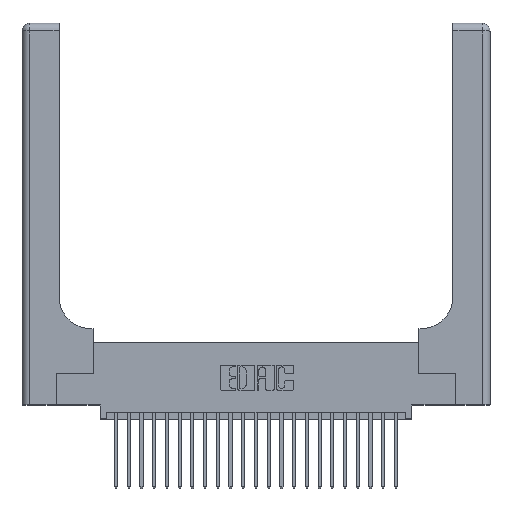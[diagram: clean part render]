
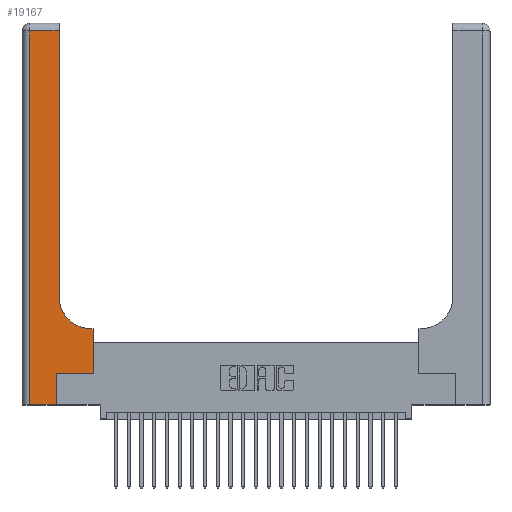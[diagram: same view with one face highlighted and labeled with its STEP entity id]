
A CAD part, top view. The second image highlights one B-rep face of the part: STEP entity #19167.
In plain terms, the highlighted planar face has unit normal (0, 0, 1).
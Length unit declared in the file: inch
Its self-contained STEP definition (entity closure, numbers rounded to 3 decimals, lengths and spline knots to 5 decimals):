
#268 = DIRECTION ( 'NONE',  ( -1., 0., 0. ) ) ;
#903 = VERTEX_POINT ( 'NONE', #4568 ) ;
#932 = ORIENTED_EDGE ( 'NONE', *, *, #19838, .T. ) ;
#1337 = CARTESIAN_POINT ( 'NONE',  ( 0.2915, 3., 0.37 ) ) ;
#1704 = EDGE_CURVE ( 'NONE', #14161, #14993, #12428, .T. ) ;
#1859 = VERTEX_POINT ( 'NONE', #20429 ) ;
#2014 = VECTOR ( 'NONE', #23446, 39.37008 ) ;
#2452 = VECTOR ( 'NONE', #6603, 39.37008 ) ;
#2461 = EDGE_CURVE ( 'NONE', #14993, #22639, #18702, .T. ) ;
#2521 = CARTESIAN_POINT ( 'NONE',  ( 0.06, 3., 0.37 ) ) ;
#3290 = ORIENTED_EDGE ( 'NONE', *, *, #21870, .T. ) ;
#3379 = DIRECTION ( 'NONE',  ( 0., 1., 0. ) ) ;
#3466 = VECTOR ( 'NONE', #22669, 39.37008 ) ;
#3483 = EDGE_CURVE ( 'NONE', #8144, #9701, #10486, .T. ) ;
#3572 = CARTESIAN_POINT ( 'NONE',  ( 0.5585, 0.25, 0.37 ) ) ;
#3951 = LINE ( 'NONE', #1337, #19370 ) ;
#4500 = VECTOR ( 'NONE', #24933, 39.37008 ) ;
#4568 = CARTESIAN_POINT ( 'NONE',  ( 0.2915, 0.85, 0.37 ) ) ;
#4932 = CARTESIAN_POINT ( 'NONE',  ( 0., 2.94, 0.37 ) ) ;
#5157 = EDGE_CURVE ( 'NONE', #17189, #1859, #8829, .T. ) ;
#6464 = DIRECTION ( 'NONE',  ( 0., 1., 0. ) ) ;
#6555 = CARTESIAN_POINT ( 'NONE',  ( 0.5585, 0.25, 0.37 ) ) ;
#6580 = FACE_OUTER_BOUND ( 'NONE', #18235, .T. ) ;
#6603 = DIRECTION ( 'NONE',  ( 0., -1., 0. ) ) ;
#7119 = VECTOR ( 'NONE', #23018, 39.37008 ) ;
#7615 = ORIENTED_EDGE ( 'NONE', *, *, #19316, .T. ) ;
#8144 = VERTEX_POINT ( 'NONE', #15929 ) ;
#8188 = CARTESIAN_POINT ( 'NONE',  ( 0.5415, 0.85, 0.37 ) ) ;
#8303 = ORIENTED_EDGE ( 'NONE', *, *, #5157, .T. ) ;
#8829 = LINE ( 'NONE', #10670, #3466 ) ;
#9701 = VERTEX_POINT ( 'NONE', #14956 ) ;
#10174 = DIRECTION ( 'NONE',  ( 1., 0., 0. ) ) ;
#10392 = PLANE ( 'NONE',  #22720 ) ;
#10486 = LINE ( 'NONE', #4932, #4500 ) ;
#10670 = CARTESIAN_POINT ( 'NONE',  ( 0., 0., 0.37 ) ) ;
#12412 = DIRECTION ( 'NONE',  ( 0., 0., -1. ) ) ;
#12428 = LINE ( 'NONE', #23324, #7119 ) ;
#12727 = VECTOR ( 'NONE', #6464, 39.37008 ) ;
#12863 = VECTOR ( 'NONE', #19005, 39.37008 ) ;
#13140 = CARTESIAN_POINT ( 'NONE',  ( 0.269, 0.25, 0.37 ) ) ;
#13488 = ORIENTED_EDGE ( 'NONE', *, *, #3483, .T. ) ;
#13822 = EDGE_CURVE ( 'NONE', #16877, #903, #24561, .T. ) ;
#14161 = VERTEX_POINT ( 'NONE', #13140 ) ;
#14956 = CARTESIAN_POINT ( 'NONE',  ( 0.06, 2.94, 0.37 ) ) ;
#14993 = VERTEX_POINT ( 'NONE', #3572 ) ;
#15753 = CARTESIAN_POINT ( 'NONE',  ( 0.5415, 0.6, 0.37 ) ) ;
#15929 = CARTESIAN_POINT ( 'NONE',  ( 0.2915, 2.94, 0.37 ) ) ;
#16051 = CARTESIAN_POINT ( 'NONE',  ( 0.5585, 0.6, 0.37 ) ) ;
#16877 = VERTEX_POINT ( 'NONE', #15753 ) ;
#17029 = CARTESIAN_POINT ( 'NONE',  ( 0.269, 0., 0.37 ) ) ;
#17189 = VERTEX_POINT ( 'NONE', #24076 ) ;
#17343 = ORIENTED_EDGE ( 'NONE', *, *, #25096, .T. ) ;
#17542 = ORIENTED_EDGE ( 'NONE', *, *, #1704, .T. ) ;
#18132 = ORIENTED_EDGE ( 'NONE', *, *, #2461, .T. ) ;
#18235 = EDGE_LOOP ( 'NONE', ( #17343, #13488, #932, #8303, #7615, #17542, #18132, #3290, #20152 ) ) ;
#18702 = LINE ( 'NONE', #6555, #12727 ) ;
#19005 = DIRECTION ( 'NONE',  ( 0., 1., 0. ) ) ;
#19149 = AXIS2_PLACEMENT_3D ( 'NONE', #8188, #22206, #10174 ) ;
#19152 = LINE ( 'NONE', #2521, #2452 ) ;
#19167 = ADVANCED_FACE ( 'NONE', ( #6580 ), #10392, .F. ) ;
#19316 = EDGE_CURVE ( 'NONE', #1859, #14161, #23452, .T. ) ;
#19370 = VECTOR ( 'NONE', #3379, 39.37008 ) ;
#19838 = EDGE_CURVE ( 'NONE', #9701, #17189, #19152, .T. ) ;
#20152 = ORIENTED_EDGE ( 'NONE', *, *, #13822, .T. ) ;
#20429 = CARTESIAN_POINT ( 'NONE',  ( 0.269, 0., 0.37 ) ) ;
#21495 = CARTESIAN_POINT ( 'NONE',  ( 0.2915, 0.6, 0.37 ) ) ;
#21870 = EDGE_CURVE ( 'NONE', #22639, #16877, #23963, .T. ) ;
#22206 = DIRECTION ( 'NONE',  ( 0., 0., -1. ) ) ;
#22639 = VERTEX_POINT ( 'NONE', #16051 ) ;
#22669 = DIRECTION ( 'NONE',  ( 1., 0., 0. ) ) ;
#22720 = AXIS2_PLACEMENT_3D ( 'NONE', #24329, #12412, #268 ) ;
#23018 = DIRECTION ( 'NONE',  ( 1., 0., 0. ) ) ;
#23324 = CARTESIAN_POINT ( 'NONE',  ( 0.269, 0.25, 0.37 ) ) ;
#23446 = DIRECTION ( 'NONE',  ( -1., 0., 0. ) ) ;
#23452 = LINE ( 'NONE', #17029, #12863 ) ;
#23963 = LINE ( 'NONE', #21495, #2014 ) ;
#24076 = CARTESIAN_POINT ( 'NONE',  ( 0.06, 0., 0.37 ) ) ;
#24329 = CARTESIAN_POINT ( 'NONE',  ( 0., 3., 0.37 ) ) ;
#24561 = CIRCLE ( 'NONE', #19149, 0.25 ) ;
#24933 = DIRECTION ( 'NONE',  ( -1., 0., 0. ) ) ;
#25096 = EDGE_CURVE ( 'NONE', #903, #8144, #3951, .T. ) ;
